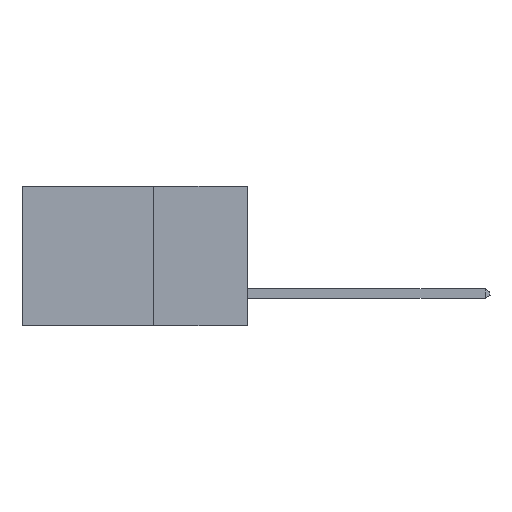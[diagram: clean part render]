
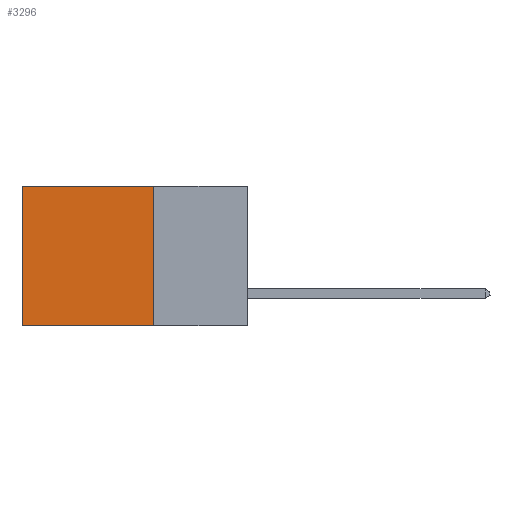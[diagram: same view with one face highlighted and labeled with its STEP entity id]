
A CAD part, left-side view. The second image highlights one B-rep face of the part: STEP entity #3296.
In plain terms, the highlighted planar face has unit normal (-1, 0, 0).
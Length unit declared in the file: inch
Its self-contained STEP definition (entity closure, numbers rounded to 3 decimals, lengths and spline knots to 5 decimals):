
#290 = CARTESIAN_POINT ( 'NONE',  ( 0.298, 0.25, 0. ) ) ;
#702 = CARTESIAN_POINT ( 'NONE',  ( 0.298, 0.25, 0. ) ) ;
#1400 = FACE_OUTER_BOUND ( 'NONE', #3150, .T. ) ;
#2602 = DIRECTION ( 'NONE',  ( 0., 0., -1. ) ) ;
#3106 = ORIENTED_EDGE ( 'NONE', *, *, #7002, .F. ) ;
#3117 = VECTOR ( 'NONE', #14581, 39.37008 ) ;
#3150 = EDGE_LOOP ( 'NONE', ( #8563, #3106, #6715, #9225 ) ) ;
#3296 = ADVANCED_FACE ( 'NONE', ( #1400 ), #13983, .F. ) ;
#3667 = VECTOR ( 'NONE', #6297, 39.37008 ) ;
#3736 = CARTESIAN_POINT ( 'NONE',  ( 0.298, 0.25, -0.37 ) ) ;
#4090 = EDGE_CURVE ( 'NONE', #6604, #12288, #7225, .T. ) ;
#4152 = DIRECTION ( 'NONE',  ( 0., 0., -1. ) ) ;
#5058 = CARTESIAN_POINT ( 'NONE',  ( 0.298, 0.6, 0. ) ) ;
#5503 = EDGE_CURVE ( 'NONE', #11697, #10729, #12298, .T. ) ;
#6072 = EDGE_CURVE ( 'NONE', #6604, #11697, #8098, .T. ) ;
#6297 = DIRECTION ( 'NONE',  ( 0., 0., -1. ) ) ;
#6604 = VERTEX_POINT ( 'NONE', #11405 ) ;
#6715 = ORIENTED_EDGE ( 'NONE', *, *, #4090, .F. ) ;
#7002 = EDGE_CURVE ( 'NONE', #12288, #10729, #12303, .T. ) ;
#7225 = LINE ( 'NONE', #702, #3667 ) ;
#7611 = CARTESIAN_POINT ( 'NONE',  ( 0.298, 0.6, 0. ) ) ;
#7932 = VECTOR ( 'NONE', #14276, 39.37008 ) ;
#8098 = LINE ( 'NONE', #13076, #7932 ) ;
#8272 = DIRECTION ( 'NONE',  ( 1., 0., 0. ) ) ;
#8563 = ORIENTED_EDGE ( 'NONE', *, *, #5503, .T. ) ;
#9225 = ORIENTED_EDGE ( 'NONE', *, *, #6072, .T. ) ;
#9588 = AXIS2_PLACEMENT_3D ( 'NONE', #290, #8272, #2602 ) ;
#10729 = VERTEX_POINT ( 'NONE', #10834 ) ;
#10834 = CARTESIAN_POINT ( 'NONE',  ( 0.298, 0.6, -0.37 ) ) ;
#11405 = CARTESIAN_POINT ( 'NONE',  ( 0.298, 0.25, 0. ) ) ;
#11697 = VERTEX_POINT ( 'NONE', #5058 ) ;
#12288 = VERTEX_POINT ( 'NONE', #3736 ) ;
#12298 = LINE ( 'NONE', #7611, #13524 ) ;
#12303 = LINE ( 'NONE', #13405, #3117 ) ;
#13076 = CARTESIAN_POINT ( 'NONE',  ( 0.298, 0.25, 0. ) ) ;
#13405 = CARTESIAN_POINT ( 'NONE',  ( 0.298, 0.25, -0.37 ) ) ;
#13524 = VECTOR ( 'NONE', #4152, 39.37008 ) ;
#13983 = PLANE ( 'NONE',  #9588 ) ;
#14276 = DIRECTION ( 'NONE',  ( 0., 1., 0. ) ) ;
#14581 = DIRECTION ( 'NONE',  ( 0., 1., 0. ) ) ;
